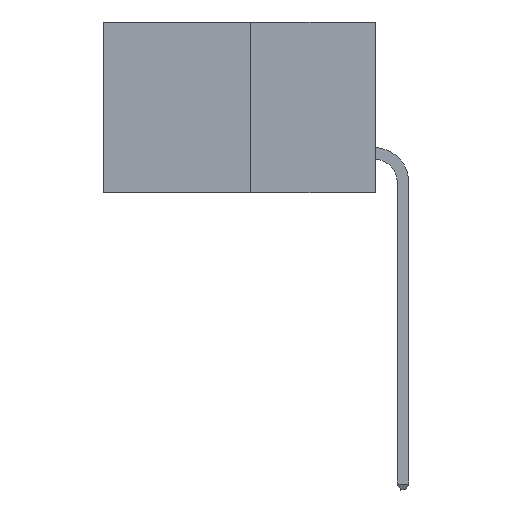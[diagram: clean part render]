
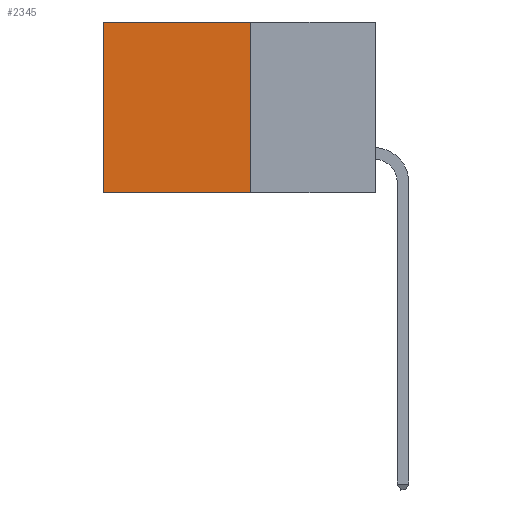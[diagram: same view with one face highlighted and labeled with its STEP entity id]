
A CAD part, left-side view. The second image highlights one B-rep face of the part: STEP entity #2345.
In plain terms, the highlighted planar face has unit normal (-1, 0, 0).
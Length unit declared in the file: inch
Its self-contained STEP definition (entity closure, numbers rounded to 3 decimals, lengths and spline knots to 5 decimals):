
#34 = EDGE_CURVE ( 'NONE', #10072, #13600, #6524, .T. ) ;
#846 = EDGE_LOOP ( 'NONE', ( #1959, #5116, #10995, #2323 ) ) ;
#1959 = ORIENTED_EDGE ( 'NONE', *, *, #12039, .T. ) ;
#2323 = ORIENTED_EDGE ( 'NONE', *, *, #10483, .T. ) ;
#2345 = ADVANCED_FACE ( 'NONE', ( #6276 ), #6732, .F. ) ;
#2530 = LINE ( 'NONE', #14340, #11187 ) ;
#3045 = VECTOR ( 'NONE', #8304, 39.37008 ) ;
#3427 = DIRECTION ( 'NONE',  ( 0., 1., 0. ) ) ;
#3441 = LINE ( 'NONE', #7190, #3045 ) ;
#3684 = DIRECTION ( 'NONE',  ( 0., 1., 0. ) ) ;
#3868 = CARTESIAN_POINT ( 'NONE',  ( 0.277, 0.27, -0.37 ) ) ;
#4409 = DIRECTION ( 'NONE',  ( 0., 0., -1. ) ) ;
#4693 = AXIS2_PLACEMENT_3D ( 'NONE', #3868, #7010, #4409 ) ;
#5116 = ORIENTED_EDGE ( 'NONE', *, *, #6671, .F. ) ;
#5425 = CARTESIAN_POINT ( 'NONE',  ( 0.277, 0.59, 0. ) ) ;
#5608 = VERTEX_POINT ( 'NONE', #10837 ) ;
#5617 = CARTESIAN_POINT ( 'NONE',  ( 0.277, 0.27, -0.37 ) ) ;
#6160 = VECTOR ( 'NONE', #12584, 39.37008 ) ;
#6276 = FACE_OUTER_BOUND ( 'NONE', #846, .T. ) ;
#6400 = CARTESIAN_POINT ( 'NONE',  ( 0.277, 0.27, 0. ) ) ;
#6524 = LINE ( 'NONE', #11140, #6160 ) ;
#6671 = EDGE_CURVE ( 'NONE', #13600, #5608, #13025, .T. ) ;
#6732 = PLANE ( 'NONE',  #4693 ) ;
#7010 = DIRECTION ( 'NONE',  ( 1., 0., 0. ) ) ;
#7190 = CARTESIAN_POINT ( 'NONE',  ( 0.277, 0.59, -0.37 ) ) ;
#7380 = VECTOR ( 'NONE', #3684, 39.37008 ) ;
#8304 = DIRECTION ( 'NONE',  ( 0., 0., -1. ) ) ;
#8438 = VERTEX_POINT ( 'NONE', #5425 ) ;
#10072 = VERTEX_POINT ( 'NONE', #6400 ) ;
#10483 = EDGE_CURVE ( 'NONE', #10072, #8438, #2530, .T. ) ;
#10837 = CARTESIAN_POINT ( 'NONE',  ( 0.277, 0.59, -0.37 ) ) ;
#10995 = ORIENTED_EDGE ( 'NONE', *, *, #34, .F. ) ;
#11140 = CARTESIAN_POINT ( 'NONE',  ( 0.277, 0.27, -0.37 ) ) ;
#11187 = VECTOR ( 'NONE', #3427, 39.37008 ) ;
#12039 = EDGE_CURVE ( 'NONE', #8438, #5608, #3441, .T. ) ;
#12584 = DIRECTION ( 'NONE',  ( 0., 0., -1. ) ) ;
#13025 = LINE ( 'NONE', #13482, #7380 ) ;
#13482 = CARTESIAN_POINT ( 'NONE',  ( 0.277, 0.27, -0.37 ) ) ;
#13600 = VERTEX_POINT ( 'NONE', #5617 ) ;
#14340 = CARTESIAN_POINT ( 'NONE',  ( 0.277, 0.27, 0. ) ) ;
